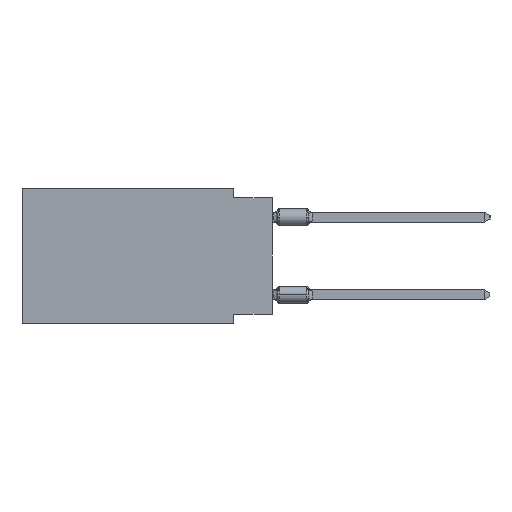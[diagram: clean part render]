
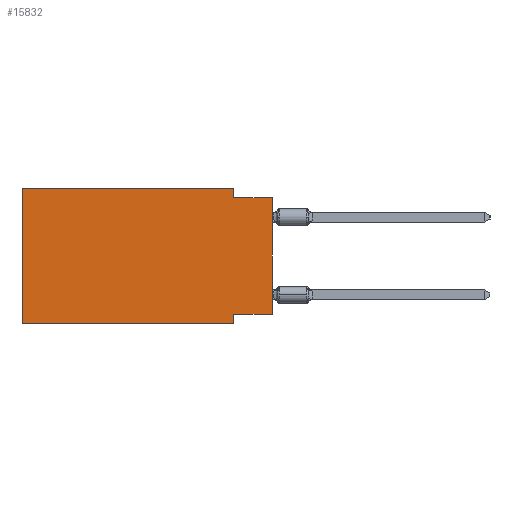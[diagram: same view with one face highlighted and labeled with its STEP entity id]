
A CAD part, left-side view. The second image highlights one B-rep face of the part: STEP entity #15832.
In plain terms, the highlighted planar face has unit normal (-1, 0, 0).
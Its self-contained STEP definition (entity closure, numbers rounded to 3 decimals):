
#148 = CARTESIAN_POINT ( 'NONE',  ( 0., 2.54, 0. ) ) ;
#1454 = DIRECTION ( 'NONE',  ( 0., 0., 1. ) ) ;
#2035 = ORIENTED_EDGE ( 'NONE', *, *, #5019, .F. ) ;
#2113 = VECTOR ( 'NONE', #44814, 1000. ) ;
#2139 = DIRECTION ( 'NONE',  ( 0., 0., 1. ) ) ;
#2348 = CARTESIAN_POINT ( 'NONE',  ( 0., 2.54, -8.89 ) ) ;
#2453 = ORIENTED_EDGE ( 'NONE', *, *, #20655, .F. ) ;
#3702 = CARTESIAN_POINT ( 'NONE',  ( 0., 0., -0.635 ) ) ;
#3729 = ORIENTED_EDGE ( 'NONE', *, *, #27655, .T. ) ;
#4209 = CARTESIAN_POINT ( 'NONE',  ( 0., 0., 0. ) ) ;
#5019 = EDGE_CURVE ( 'NONE', #16455, #41567, #33346, .T. ) ;
#6109 = EDGE_CURVE ( 'NONE', #13470, #16455, #33459, .T. ) ;
#6452 = DIRECTION ( 'NONE',  ( 1., 0., 0. ) ) ;
#7150 = LINE ( 'NONE', #13138, #21904 ) ;
#7495 = EDGE_CURVE ( 'NONE', #38651, #18356, #39632, .T. ) ;
#8398 = ORIENTED_EDGE ( 'NONE', *, *, #6109, .F. ) ;
#8988 = CARTESIAN_POINT ( 'NONE',  ( 0., 16.383, 0. ) ) ;
#9685 = DIRECTION ( 'NONE',  ( 0., 1., 0. ) ) ;
#9809 = CARTESIAN_POINT ( 'NONE',  ( 0., 2.54, -8.89 ) ) ;
#10344 = DIRECTION ( 'NONE',  ( 0., 0., -1. ) ) ;
#11339 = VERTEX_POINT ( 'NONE', #38897 ) ;
#11377 = EDGE_CURVE ( 'NONE', #38059, #18356, #14001, .T. ) ;
#11969 = VECTOR ( 'NONE', #2139, 1000. ) ;
#12727 = LINE ( 'NONE', #23001, #38613 ) ;
#13138 = CARTESIAN_POINT ( 'NONE',  ( 0., 0., -8.255 ) ) ;
#13470 = VERTEX_POINT ( 'NONE', #26307 ) ;
#14001 = LINE ( 'NONE', #3702, #14413 ) ;
#14231 = DIRECTION ( 'NONE',  ( 0., -1., 0. ) ) ;
#14413 = VECTOR ( 'NONE', #14231, 1000. ) ;
#14706 = LINE ( 'NONE', #42589, #16426 ) ;
#15832 = ADVANCED_FACE ( 'NONE', ( #23599 ), #27941, .F. ) ;
#16426 = VECTOR ( 'NONE', #21330, 1000. ) ;
#16455 = VERTEX_POINT ( 'NONE', #28997 ) ;
#16918 = LINE ( 'NONE', #9809, #2113 ) ;
#17394 = EDGE_CURVE ( 'NONE', #38651, #11339, #7150, .T. ) ;
#18301 = ORIENTED_EDGE ( 'NONE', *, *, #11377, .F. ) ;
#18356 = VERTEX_POINT ( 'NONE', #26166 ) ;
#19002 = AXIS2_PLACEMENT_3D ( 'NONE', #23827, #6452, #10344 ) ;
#20655 = EDGE_CURVE ( 'NONE', #11339, #36897, #16918, .T. ) ;
#20822 = CARTESIAN_POINT ( 'NONE',  ( 0., 0., -8.255 ) ) ;
#21330 = DIRECTION ( 'NONE',  ( 0., -1., 0. ) ) ;
#21904 = VECTOR ( 'NONE', #9685, 1000. ) ;
#23001 = CARTESIAN_POINT ( 'NONE',  ( 0., 2.54, 0. ) ) ;
#23306 = ORIENTED_EDGE ( 'NONE', *, *, #7495, .T. ) ;
#23599 = FACE_OUTER_BOUND ( 'NONE', #24041, .T. ) ;
#23827 = CARTESIAN_POINT ( 'NONE',  ( 0., 16.383, 0. ) ) ;
#24041 = EDGE_LOOP ( 'NONE', ( #23306, #18301, #43403, #2035, #8398, #3729, #2453, #37412 ) ) ;
#26166 = CARTESIAN_POINT ( 'NONE',  ( 0., 0., -0.635 ) ) ;
#26307 = CARTESIAN_POINT ( 'NONE',  ( 0., 16.383, -8.89 ) ) ;
#26927 = CARTESIAN_POINT ( 'NONE',  ( 0., 16.383, 0. ) ) ;
#27268 = CARTESIAN_POINT ( 'NONE',  ( 0., 2.54, -0.635 ) ) ;
#27655 = EDGE_CURVE ( 'NONE', #13470, #36897, #14706, .T. ) ;
#27941 = PLANE ( 'NONE',  #19002 ) ;
#28997 = CARTESIAN_POINT ( 'NONE',  ( 0., 16.383, 0. ) ) ;
#33062 = DIRECTION ( 'NONE',  ( 0., 0., -1. ) ) ;
#33346 = LINE ( 'NONE', #26927, #39638 ) ;
#33459 = LINE ( 'NONE', #8988, #11969 ) ;
#34013 = DIRECTION ( 'NONE',  ( 0., -1., 0. ) ) ;
#36897 = VERTEX_POINT ( 'NONE', #2348 ) ;
#37412 = ORIENTED_EDGE ( 'NONE', *, *, #17394, .F. ) ;
#38059 = VERTEX_POINT ( 'NONE', #27268 ) ;
#38613 = VECTOR ( 'NONE', #33062, 1000. ) ;
#38651 = VERTEX_POINT ( 'NONE', #20822 ) ;
#38897 = CARTESIAN_POINT ( 'NONE',  ( 0., 2.54, -8.255 ) ) ;
#39391 = EDGE_CURVE ( 'NONE', #41567, #38059, #12727, .T. ) ;
#39632 = LINE ( 'NONE', #4209, #40583 ) ;
#39638 = VECTOR ( 'NONE', #34013, 1000. ) ;
#40583 = VECTOR ( 'NONE', #1454, 1000. ) ;
#41567 = VERTEX_POINT ( 'NONE', #148 ) ;
#42589 = CARTESIAN_POINT ( 'NONE',  ( 0., 16.383, -8.89 ) ) ;
#43403 = ORIENTED_EDGE ( 'NONE', *, *, #39391, .F. ) ;
#44814 = DIRECTION ( 'NONE',  ( 0., 0., -1. ) ) ;
